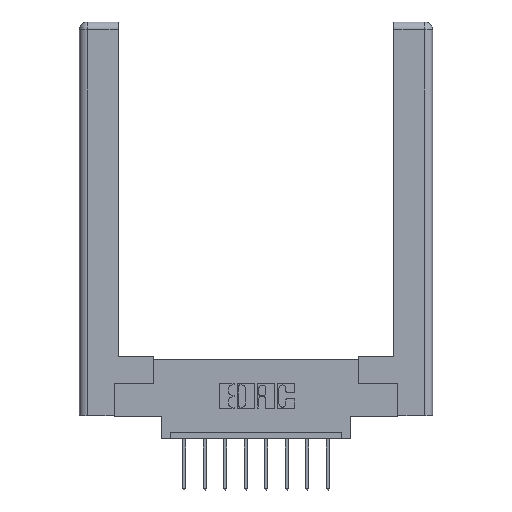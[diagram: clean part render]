
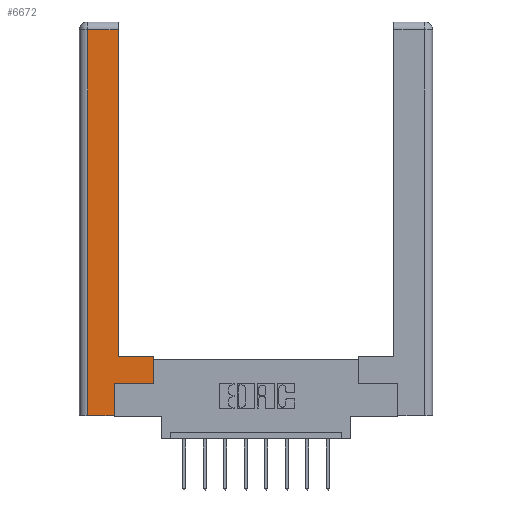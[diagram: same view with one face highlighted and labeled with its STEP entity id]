
A CAD part, top view. The second image highlights one B-rep face of the part: STEP entity #6672.
In plain terms, the highlighted planar face has unit normal (0, 0, 1).
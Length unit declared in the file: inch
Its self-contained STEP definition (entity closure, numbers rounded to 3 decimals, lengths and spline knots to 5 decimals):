
#45 = CARTESIAN_POINT ( 'NONE',  ( 0.295, 3., 0. ) ) ;
#100 = DIRECTION ( 'NONE',  ( -1., 0., 0. ) ) ;
#163 = ORIENTED_EDGE ( 'NONE', *, *, #4887, .T. ) ;
#280 = CARTESIAN_POINT ( 'NONE',  ( 0.0615, 2.94, 0. ) ) ;
#443 = FACE_OUTER_BOUND ( 'NONE', #11156, .T. ) ;
#657 = VECTOR ( 'NONE', #10917, 39.37008 ) ;
#883 = DIRECTION ( 'NONE',  ( 0., 1., 0. ) ) ;
#1006 = DIRECTION ( 'NONE',  ( 1., 0., 0. ) ) ;
#1204 = ORIENTED_EDGE ( 'NONE', *, *, #13009, .T. ) ;
#1491 = DIRECTION ( 'NONE',  ( 1., 0., 0. ) ) ;
#1801 = EDGE_CURVE ( 'NONE', #10683, #4073, #9621, .T. ) ;
#1840 = CARTESIAN_POINT ( 'NONE',  ( 0.565, 0.45, 0. ) ) ;
#2057 = VERTEX_POINT ( 'NONE', #5089 ) ;
#2821 = CARTESIAN_POINT ( 'NONE',  ( 0.565, 0.245, 0. ) ) ;
#3178 = VECTOR ( 'NONE', #1491, 39.37008 ) ;
#3321 = DIRECTION ( 'NONE',  ( 0., 0., -1. ) ) ;
#3491 = LINE ( 'NONE', #3847, #12117 ) ;
#3506 = VECTOR ( 'NONE', #10857, 39.37008 ) ;
#3560 = ORIENTED_EDGE ( 'NONE', *, *, #8702, .T. ) ;
#3804 = CARTESIAN_POINT ( 'NONE',  ( 0.0615, 0., 0. ) ) ;
#3833 = LINE ( 'NONE', #7765, #3506 ) ;
#3847 = CARTESIAN_POINT ( 'NONE',  ( 0.565, 0.245, 0. ) ) ;
#4073 = VERTEX_POINT ( 'NONE', #5570 ) ;
#4199 = VERTEX_POINT ( 'NONE', #9910 ) ;
#4370 = VERTEX_POINT ( 'NONE', #280 ) ;
#4425 = EDGE_CURVE ( 'NONE', #4073, #2057, #7291, .T. ) ;
#4887 = EDGE_CURVE ( 'NONE', #4370, #10683, #6299, .T. ) ;
#4937 = ORIENTED_EDGE ( 'NONE', *, *, #8059, .T. ) ;
#5089 = CARTESIAN_POINT ( 'NONE',  ( 0.265, 0.245, 0. ) ) ;
#5502 = CARTESIAN_POINT ( 'NONE',  ( 0.265, 0., 0. ) ) ;
#5570 = CARTESIAN_POINT ( 'NONE',  ( 0.265, 0., 0. ) ) ;
#5935 = AXIS2_PLACEMENT_3D ( 'NONE', #11479, #3321, #9393 ) ;
#5964 = ORIENTED_EDGE ( 'NONE', *, *, #1801, .T. ) ;
#6199 = CARTESIAN_POINT ( 'NONE',  ( 0.295, 0.45, 0. ) ) ;
#6299 = LINE ( 'NONE', #3804, #657 ) ;
#6506 = VERTEX_POINT ( 'NONE', #7315 ) ;
#6672 = ADVANCED_FACE ( 'NONE', ( #443 ), #9532, .F. ) ;
#6926 = EDGE_CURVE ( 'NONE', #8657, #4199, #11873, .T. ) ;
#7101 = DIRECTION ( 'NONE',  ( 0., 1., 0. ) ) ;
#7291 = LINE ( 'NONE', #11543, #8100 ) ;
#7315 = CARTESIAN_POINT ( 'NONE',  ( 0.295, 2.94, 0. ) ) ;
#7511 = VECTOR ( 'NONE', #100, 39.37008 ) ;
#7765 = CARTESIAN_POINT ( 'NONE',  ( 0.0615, 2.94, 0. ) ) ;
#8059 = EDGE_CURVE ( 'NONE', #4199, #11500, #11522, .T. ) ;
#8100 = VECTOR ( 'NONE', #12582, 39.37008 ) ;
#8657 = VERTEX_POINT ( 'NONE', #2821 ) ;
#8702 = EDGE_CURVE ( 'NONE', #2057, #8657, #3491, .T. ) ;
#9393 = DIRECTION ( 'NONE',  ( -1., 0., 0. ) ) ;
#9428 = EDGE_CURVE ( 'NONE', #6506, #4370, #3833, .T. ) ;
#9532 = PLANE ( 'NONE',  #5935 ) ;
#9621 = LINE ( 'NONE', #5502, #3178 ) ;
#9653 = LINE ( 'NONE', #45, #12783 ) ;
#9830 = ORIENTED_EDGE ( 'NONE', *, *, #9428, .T. ) ;
#9910 = CARTESIAN_POINT ( 'NONE',  ( 0.565, 0.45, 0. ) ) ;
#10177 = CARTESIAN_POINT ( 'NONE',  ( 0.295, 0.45, 0. ) ) ;
#10393 = CARTESIAN_POINT ( 'NONE',  ( 0.0615, 0., 0. ) ) ;
#10683 = VERTEX_POINT ( 'NONE', #10393 ) ;
#10715 = ORIENTED_EDGE ( 'NONE', *, *, #6926, .T. ) ;
#10857 = DIRECTION ( 'NONE',  ( -1., 0., 0. ) ) ;
#10917 = DIRECTION ( 'NONE',  ( 0., -1., 0. ) ) ;
#11156 = EDGE_LOOP ( 'NONE', ( #1204, #9830, #163, #5964, #11531, #3560, #10715, #4937 ) ) ;
#11479 = CARTESIAN_POINT ( 'NONE',  ( 0., 0., 0. ) ) ;
#11500 = VERTEX_POINT ( 'NONE', #10177 ) ;
#11522 = LINE ( 'NONE', #6199, #7511 ) ;
#11531 = ORIENTED_EDGE ( 'NONE', *, *, #4425, .T. ) ;
#11543 = CARTESIAN_POINT ( 'NONE',  ( 0.265, 0.245, 0. ) ) ;
#11873 = LINE ( 'NONE', #1840, #12487 ) ;
#12117 = VECTOR ( 'NONE', #1006, 39.37008 ) ;
#12487 = VECTOR ( 'NONE', #883, 39.37008 ) ;
#12582 = DIRECTION ( 'NONE',  ( 0., 1., 0. ) ) ;
#12783 = VECTOR ( 'NONE', #7101, 39.37008 ) ;
#13009 = EDGE_CURVE ( 'NONE', #11500, #6506, #9653, .T. ) ;
